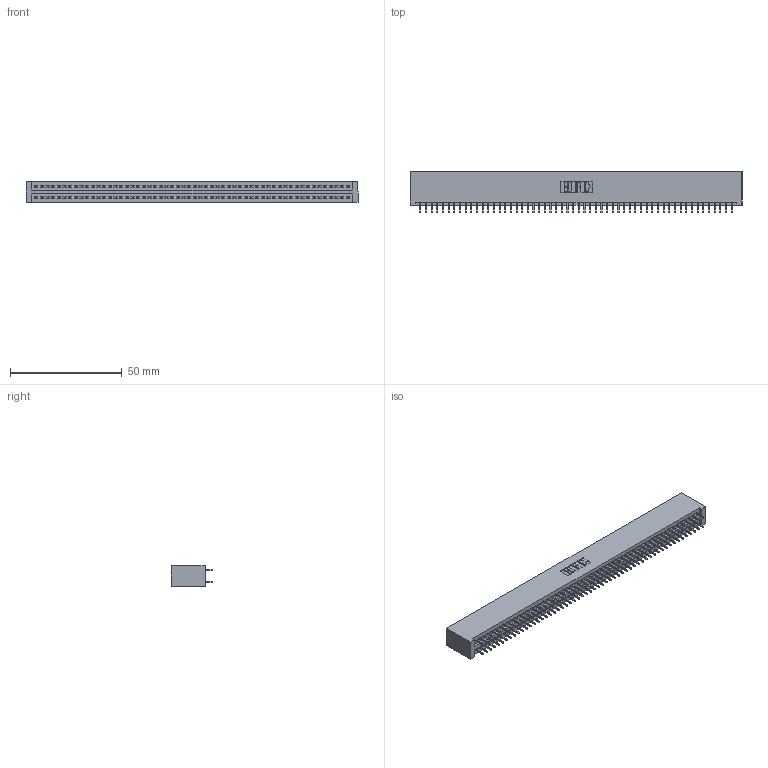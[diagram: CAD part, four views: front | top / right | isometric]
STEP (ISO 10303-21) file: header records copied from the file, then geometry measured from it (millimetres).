
FILE_DESCRIPTION (( 'STEP AP203' ), '1' );
FILE_NAME ('395-112-525-201.STEP', '2020-09-25T19:28:17', ( '' ), ( '' ), 'SwSTEP 2.0', 'SolidWorks 2020', '' );
FILE_SCHEMA (( 'CONFIG_CONTROL_DESIGN' ));
Length unit declared in the file: inch
Products named in the file (3): 345-292-001_345-293-125; 395-112-525-201; 345 Part_No Mounting Lugs
Assembly tree (113 placements, depth 2):
  395-112-525-201
    345 Part_No Mounting Lugs
    345-292-001_345-293-125  x112
Bounding box: 148.84 x 18.72 x 9.4 mm (x, y, z)
Volume: 15020.4 mm3; surface area: 22221.5 mm2
Topology: 113 solids, 113 shells, 6166 faces, 17453 edges, 11186 vertices
Faces by surface type: plane 4444, cylinder 1722
Entity records: 41851 total; most frequent: CARTESIAN_POINT 7000, ORIENTED_EDGE 6934, DIRECTION 6151, EDGE_CURVE 3467, LINE 3123, VECTOR 3123, VERTEX_POINT 2306, AXIS2_PLACEMENT_3D 1514
